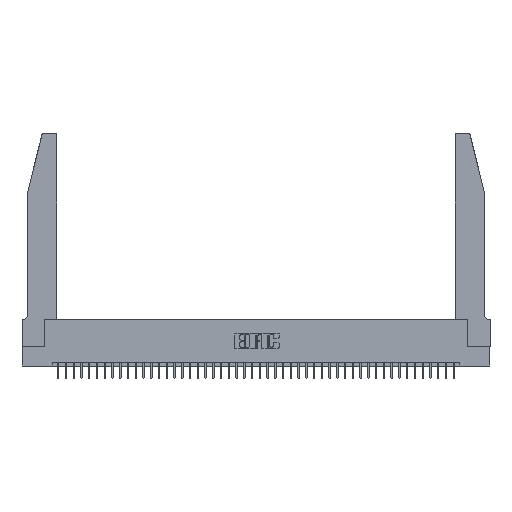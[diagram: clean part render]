
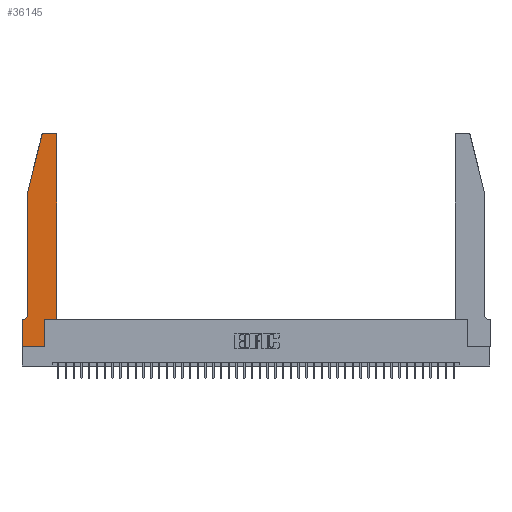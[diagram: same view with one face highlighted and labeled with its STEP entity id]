
A CAD part, top view. The second image highlights one B-rep face of the part: STEP entity #36145.
In plain terms, the highlighted planar face has unit normal (0, 0, 1).
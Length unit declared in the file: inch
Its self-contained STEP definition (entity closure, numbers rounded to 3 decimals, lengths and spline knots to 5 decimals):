
#39 = CARTESIAN_POINT ( 'NONE',  ( 0.25487, 2.72718, 0.37 ) ) ;
#286 = EDGE_CURVE ( 'NONE', #16809, #10562, #3333, .T. ) ;
#864 = DIRECTION ( 'NONE',  ( 0., -1., 0. ) ) ;
#1812 = DIRECTION ( 'NONE',  ( 0., 0., 1. ) ) ;
#1998 = AXIS2_PLACEMENT_3D ( 'NONE', #17694, #41349, #21152 ) ;
#2662 = LINE ( 'NONE', #19239, #37993 ) ;
#3333 = CIRCLE ( 'NONE', #1998, 0.07 ) ;
#3372 = CARTESIAN_POINT ( 'NONE',  ( 0., 0.35, 0.37 ) ) ;
#3655 = CARTESIAN_POINT ( 'NONE',  ( 0.4205, 2.75, 0.37 ) ) ;
#4065 = CARTESIAN_POINT ( 'NONE',  ( 0.4505, 0.35, 0.37 ) ) ;
#4110 = VERTEX_POINT ( 'NONE', #19731 ) ;
#4639 = CARTESIAN_POINT ( 'NONE',  ( 0.0755, 0.35, 0.37 ) ) ;
#4648 = ORIENTED_EDGE ( 'NONE', *, *, #7338, .T. ) ;
#5060 = VERTEX_POINT ( 'NONE', #41104 ) ;
#5206 = EDGE_CURVE ( 'NONE', #15467, #41717, #37167, .T. ) ;
#5564 = DIRECTION ( 'NONE',  ( 0., -1., 0. ) ) ;
#5793 = EDGE_CURVE ( 'NONE', #21103, #25071, #15898, .T. ) ;
#5809 = AXIS2_PLACEMENT_3D ( 'NONE', #3372, #17306, #40959 ) ;
#6892 = VERTEX_POINT ( 'NONE', #3655 ) ;
#7338 = EDGE_CURVE ( 'NONE', #9374, #21103, #20104, .T. ) ;
#7579 = VECTOR ( 'NONE', #35433, 39.37008 ) ;
#8440 = LINE ( 'NONE', #4639, #36660 ) ;
#9374 = VERTEX_POINT ( 'NONE', #12905 ) ;
#9561 = DIRECTION ( 'NONE',  ( 0., 0., 1. ) ) ;
#9652 = CARTESIAN_POINT ( 'NONE',  ( 0.0055, 0.35, 0.37 ) ) ;
#10054 = VECTOR ( 'NONE', #864, 39.37008 ) ;
#10562 = VERTEX_POINT ( 'NONE', #9652 ) ;
#11015 = VECTOR ( 'NONE', #26819, 39.37008 ) ;
#11301 = CARTESIAN_POINT ( 'NONE',  ( 0., 0., 0.37 ) ) ;
#11474 = AXIS2_PLACEMENT_3D ( 'NONE', #29996, #9561, #33378 ) ;
#11720 = ORIENTED_EDGE ( 'NONE', *, *, #20439, .T. ) ;
#12905 = CARTESIAN_POINT ( 'NONE',  ( 0.2865, 0., 0.37 ) ) ;
#13036 = DIRECTION ( 'NONE',  ( -1., 0., 0. ) ) ;
#13198 = CARTESIAN_POINT ( 'NONE',  ( 0.2865, 0.35, 0.37 ) ) ;
#15467 = VERTEX_POINT ( 'NONE', #35166 ) ;
#15898 = LINE ( 'NONE', #4065, #33941 ) ;
#16197 = EDGE_CURVE ( 'NONE', #10562, #15467, #8440, .T. ) ;
#16241 = LINE ( 'NONE', #40040, #33228 ) ;
#16739 = LINE ( 'NONE', #32026, #7579 ) ;
#16809 = VERTEX_POINT ( 'NONE', #31664 ) ;
#17099 = ORIENTED_EDGE ( 'NONE', *, *, #286, .T. ) ;
#17103 = LINE ( 'NONE', #29955, #32995 ) ;
#17306 = DIRECTION ( 'NONE',  ( 0., 0., 1. ) ) ;
#17317 = CARTESIAN_POINT ( 'NONE',  ( 0., 0., 0.37 ) ) ;
#17606 = ORIENTED_EDGE ( 'NONE', *, *, #30891, .T. ) ;
#17694 = CARTESIAN_POINT ( 'NONE',  ( 0.0055, 0.42, 0.37 ) ) ;
#18502 = CARTESIAN_POINT ( 'NONE',  ( 0.4505, 0.35, 0.37 ) ) ;
#19239 = CARTESIAN_POINT ( 'NONE',  ( 0.0755, 2., 0.37 ) ) ;
#19731 = CARTESIAN_POINT ( 'NONE',  ( 0.284, 2.75, 0.37 ) ) ;
#20104 = LINE ( 'NONE', #13198, #11015 ) ;
#20342 = VECTOR ( 'NONE', #13036, 39.37008 ) ;
#20439 = EDGE_CURVE ( 'NONE', #25071, #42318, #16739, .T. ) ;
#20683 = CARTESIAN_POINT ( 'NONE',  ( 0.2865, 0.35, 0.37 ) ) ;
#20831 = ORIENTED_EDGE ( 'NONE', *, *, #5793, .T. ) ;
#21103 = VERTEX_POINT ( 'NONE', #20683 ) ;
#21152 = DIRECTION ( 'NONE',  ( -1., 0., 0. ) ) ;
#21388 = CIRCLE ( 'NONE', #11474, 0.03 ) ;
#22314 = FACE_OUTER_BOUND ( 'NONE', #23224, .T. ) ;
#22556 = CARTESIAN_POINT ( 'NONE',  ( 0.4205, 2.72, 0.37 ) ) ;
#22974 = ORIENTED_EDGE ( 'NONE', *, *, #33558, .T. ) ;
#23224 = EDGE_LOOP ( 'NONE', ( #34593, #32489, #23537, #29340, #17099, #43019, #40903, #22974, #4648, #20831, #11720, #17606 ) ) ;
#23537 = ORIENTED_EDGE ( 'NONE', *, *, #44019, .T. ) ;
#24733 = DIRECTION ( 'NONE',  ( 1., 0., 0. ) ) ;
#25071 = VERTEX_POINT ( 'NONE', #18502 ) ;
#25274 = DIRECTION ( 'NONE',  ( -1., 0., 0. ) ) ;
#26018 = DIRECTION ( 'NONE',  ( 1., 0., 0. ) ) ;
#26614 = DIRECTION ( 'NONE',  ( 1., 0., 0. ) ) ;
#26819 = DIRECTION ( 'NONE',  ( 0., 1., 0. ) ) ;
#29340 = ORIENTED_EDGE ( 'NONE', *, *, #30928, .T. ) ;
#29955 = CARTESIAN_POINT ( 'NONE',  ( 0., 0., 0.37 ) ) ;
#29996 = CARTESIAN_POINT ( 'NONE',  ( 0.284, 2.72, 0.37 ) ) ;
#30891 = EDGE_CURVE ( 'NONE', #42318, #6892, #40077, .T. ) ;
#30928 = EDGE_CURVE ( 'NONE', #5060, #16809, #2662, .T. ) ;
#31664 = CARTESIAN_POINT ( 'NONE',  ( 0.0755, 0.42, 0.37 ) ) ;
#32026 = CARTESIAN_POINT ( 'NONE',  ( 0.4505, 0.35, 0.37 ) ) ;
#32316 = AXIS2_PLACEMENT_3D ( 'NONE', #22556, #1812, #26018 ) ;
#32489 = ORIENTED_EDGE ( 'NONE', *, *, #41205, .T. ) ;
#32965 = EDGE_CURVE ( 'NONE', #6892, #4110, #39368, .T. ) ;
#32995 = VECTOR ( 'NONE', #26614, 39.37008 ) ;
#33228 = VECTOR ( 'NONE', #43452, 39.37008 ) ;
#33378 = DIRECTION ( 'NONE',  ( 1., 0., 0. ) ) ;
#33558 = EDGE_CURVE ( 'NONE', #41717, #9374, #17103, .T. ) ;
#33941 = VECTOR ( 'NONE', #24733, 39.37008 ) ;
#34593 = ORIENTED_EDGE ( 'NONE', *, *, #32965, .T. ) ;
#35166 = CARTESIAN_POINT ( 'NONE',  ( 0., 0.35, 0.37 ) ) ;
#35433 = DIRECTION ( 'NONE',  ( 0., 1., 0. ) ) ;
#36145 = ADVANCED_FACE ( 'NONE', ( #22314 ), #37590, .T. ) ;
#36660 = VECTOR ( 'NONE', #25274, 39.37008 ) ;
#36772 = CARTESIAN_POINT ( 'NONE',  ( 0.2605, 2.75, 0.37 ) ) ;
#37167 = LINE ( 'NONE', #11301, #10054 ) ;
#37590 = PLANE ( 'NONE',  #5809 ) ;
#37993 = VECTOR ( 'NONE', #5564, 39.37008 ) ;
#38844 = VERTEX_POINT ( 'NONE', #39 ) ;
#39368 = LINE ( 'NONE', #36772, #20342 ) ;
#40040 = CARTESIAN_POINT ( 'NONE',  ( 0.0755, 2., 0.37 ) ) ;
#40077 = CIRCLE ( 'NONE', #32316, 0.03 ) ;
#40635 = CARTESIAN_POINT ( 'NONE',  ( 0.4505, 2.72, 0.37 ) ) ;
#40903 = ORIENTED_EDGE ( 'NONE', *, *, #5206, .T. ) ;
#40959 = DIRECTION ( 'NONE',  ( 1., 0., 0. ) ) ;
#41104 = CARTESIAN_POINT ( 'NONE',  ( 0.0755, 2., 0.37 ) ) ;
#41205 = EDGE_CURVE ( 'NONE', #4110, #38844, #21388, .T. ) ;
#41349 = DIRECTION ( 'NONE',  ( 0., 0., -1. ) ) ;
#41717 = VERTEX_POINT ( 'NONE', #17317 ) ;
#42318 = VERTEX_POINT ( 'NONE', #40635 ) ;
#43019 = ORIENTED_EDGE ( 'NONE', *, *, #16197, .T. ) ;
#43452 = DIRECTION ( 'NONE',  ( -0.239, -0.971, 0. ) ) ;
#44019 = EDGE_CURVE ( 'NONE', #38844, #5060, #16241, .T. ) ;
